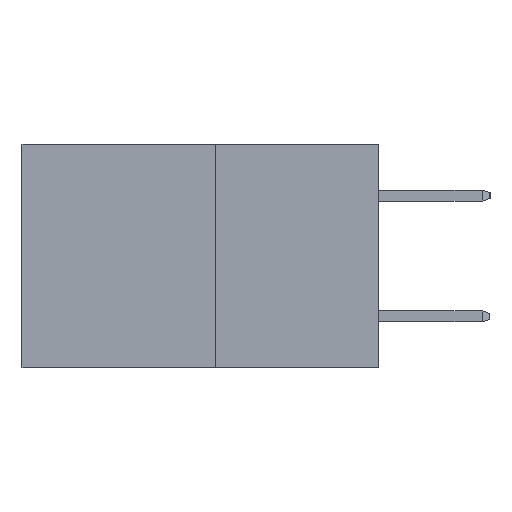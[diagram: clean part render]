
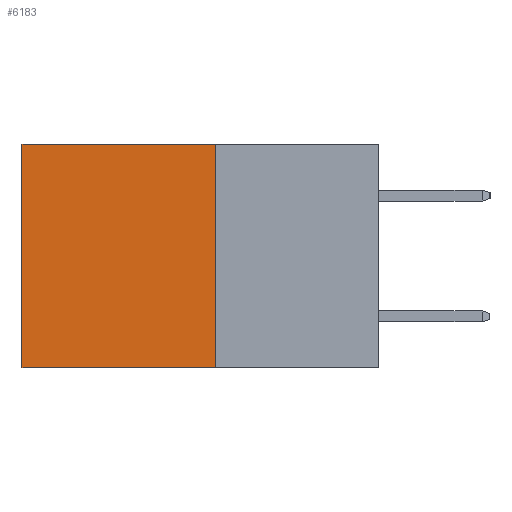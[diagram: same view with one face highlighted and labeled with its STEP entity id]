
A CAD part, left-side view. The second image highlights one B-rep face of the part: STEP entity #6183.
In plain terms, the highlighted planar face has unit normal (-1, 0, 0).
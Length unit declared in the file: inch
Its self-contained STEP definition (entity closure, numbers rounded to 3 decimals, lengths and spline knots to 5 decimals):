
#181 = DIRECTION ( 'NONE',  ( 0., 0., -1. ) ) ;
#307 = LINE ( 'NONE', #14247, #14311 ) ;
#468 = VECTOR ( 'NONE', #4605, 39.37008 ) ;
#3148 = ORIENTED_EDGE ( 'NONE', *, *, #4464, .F. ) ;
#3283 = EDGE_CURVE ( 'NONE', #11922, #5047, #307, .T. ) ;
#3329 = VERTEX_POINT ( 'NONE', #13430 ) ;
#3878 = VECTOR ( 'NONE', #6757, 39.37008 ) ;
#4464 = EDGE_CURVE ( 'NONE', #3329, #15537, #11357, .T. ) ;
#4605 = DIRECTION ( 'NONE',  ( 0., 1., 0. ) ) ;
#4770 = CARTESIAN_POINT ( 'NONE',  ( 0.277, 0.59, 0. ) ) ;
#5047 = VERTEX_POINT ( 'NONE', #4770 ) ;
#5173 = ORIENTED_EDGE ( 'NONE', *, *, #16423, .F. ) ;
#5265 = CARTESIAN_POINT ( 'NONE',  ( 0.277, 0.27, -0.37 ) ) ;
#5549 = AXIS2_PLACEMENT_3D ( 'NONE', #7184, #6826, #6800 ) ;
#6118 = CARTESIAN_POINT ( 'NONE',  ( 0.277, 0.59, -0.37 ) ) ;
#6183 = ADVANCED_FACE ( 'NONE', ( #7904 ), #7229, .F. ) ;
#6356 = EDGE_LOOP ( 'NONE', ( #10316, #3148, #5173, #8702 ) ) ;
#6647 = EDGE_CURVE ( 'NONE', #5047, #15537, #17196, .T. ) ;
#6757 = DIRECTION ( 'NONE',  ( 0., 0., -1. ) ) ;
#6800 = DIRECTION ( 'NONE',  ( 0., 0., -1. ) ) ;
#6826 = DIRECTION ( 'NONE',  ( 1., 0., 0. ) ) ;
#7184 = CARTESIAN_POINT ( 'NONE',  ( 0.277, 0.27, -0.37 ) ) ;
#7229 = PLANE ( 'NONE',  #5549 ) ;
#7904 = FACE_OUTER_BOUND ( 'NONE', #6356, .T. ) ;
#8702 = ORIENTED_EDGE ( 'NONE', *, *, #3283, .T. ) ;
#10316 = ORIENTED_EDGE ( 'NONE', *, *, #6647, .T. ) ;
#11357 = LINE ( 'NONE', #5265, #468 ) ;
#11922 = VERTEX_POINT ( 'NONE', #13955 ) ;
#13430 = CARTESIAN_POINT ( 'NONE',  ( 0.277, 0.27, -0.37 ) ) ;
#13477 = CARTESIAN_POINT ( 'NONE',  ( 0.277, 0.27, -0.37 ) ) ;
#13759 = VECTOR ( 'NONE', #181, 39.37008 ) ;
#13955 = CARTESIAN_POINT ( 'NONE',  ( 0.277, 0.27, 0. ) ) ;
#14171 = DIRECTION ( 'NONE',  ( 0., 1., 0. ) ) ;
#14247 = CARTESIAN_POINT ( 'NONE',  ( 0.277, 0.27, 0. ) ) ;
#14311 = VECTOR ( 'NONE', #14171, 39.37008 ) ;
#15049 = LINE ( 'NONE', #13477, #3878 ) ;
#15537 = VERTEX_POINT ( 'NONE', #15696 ) ;
#15696 = CARTESIAN_POINT ( 'NONE',  ( 0.277, 0.59, -0.37 ) ) ;
#16423 = EDGE_CURVE ( 'NONE', #11922, #3329, #15049, .T. ) ;
#17196 = LINE ( 'NONE', #6118, #13759 ) ;
